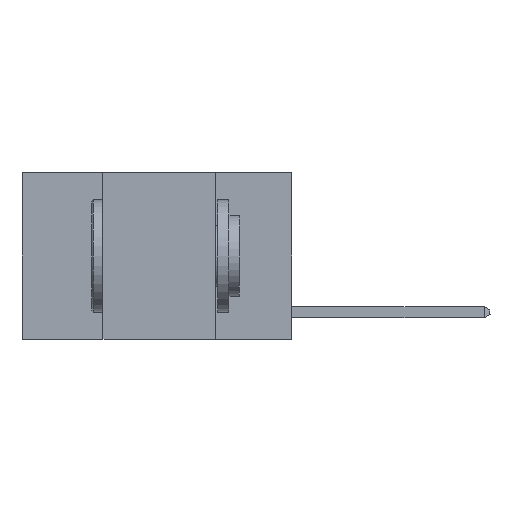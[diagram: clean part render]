
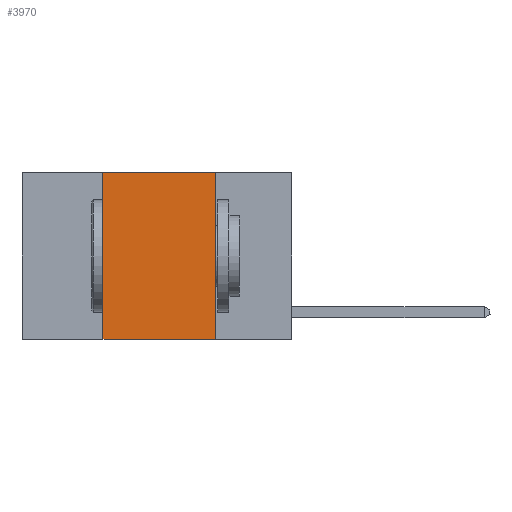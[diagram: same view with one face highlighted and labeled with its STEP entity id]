
A CAD part, left-side view. The second image highlights one B-rep face of the part: STEP entity #3970.
In plain terms, the highlighted planar face has unit normal (-1, 0, 0).
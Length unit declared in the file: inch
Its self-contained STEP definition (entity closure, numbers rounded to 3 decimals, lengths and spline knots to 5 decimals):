
#795 = VERTEX_POINT ( 'NONE', #7613 ) ;
#1009 = DIRECTION ( 'NONE',  ( 0., 0., 1. ) ) ;
#2257 = CARTESIAN_POINT ( 'NONE',  ( 0., 0.17, 0. ) ) ;
#3109 = CARTESIAN_POINT ( 'NONE',  ( 0., 0.6, 0. ) ) ;
#3128 = VERTEX_POINT ( 'NONE', #8040 ) ;
#3388 = VECTOR ( 'NONE', #11484, 39.37008 ) ;
#3541 = CARTESIAN_POINT ( 'NONE',  ( 0., 0.6, 0. ) ) ;
#3970 = ADVANCED_FACE ( 'NONE', ( #9713 ), #4510, .F. ) ;
#4170 = ORIENTED_EDGE ( 'NONE', *, *, #9298, .T. ) ;
#4510 = PLANE ( 'NONE',  #6980 ) ;
#4902 = VERTEX_POINT ( 'NONE', #6305 ) ;
#5471 = VECTOR ( 'NONE', #7393, 39.37008 ) ;
#6305 = CARTESIAN_POINT ( 'NONE',  ( 0., 0.42, 0. ) ) ;
#6980 = AXIS2_PLACEMENT_3D ( 'NONE', #3109, #11218, #14520 ) ;
#7393 = DIRECTION ( 'NONE',  ( 0., -1., 0. ) ) ;
#7411 = VECTOR ( 'NONE', #15067, 39.37008 ) ;
#7613 = CARTESIAN_POINT ( 'NONE',  ( 0., 0.17, -0.37 ) ) ;
#8040 = CARTESIAN_POINT ( 'NONE',  ( 0., 0.42, -0.37 ) ) ;
#9298 = EDGE_CURVE ( 'NONE', #3128, #795, #10453, .T. ) ;
#9713 = FACE_OUTER_BOUND ( 'NONE', #15528, .T. ) ;
#10453 = LINE ( 'NONE', #13846, #5471 ) ;
#10499 = LINE ( 'NONE', #2257, #7411 ) ;
#11218 = DIRECTION ( 'NONE',  ( 1., 0., 0. ) ) ;
#11484 = DIRECTION ( 'NONE',  ( 0., -1., 0. ) ) ;
#12625 = CARTESIAN_POINT ( 'NONE',  ( 0., 0.42, 0. ) ) ;
#13846 = CARTESIAN_POINT ( 'NONE',  ( 0., 0.6, -0.37 ) ) ;
#13991 = VERTEX_POINT ( 'NONE', #15413 ) ;
#14520 = DIRECTION ( 'NONE',  ( 0., 0., -1. ) ) ;
#15067 = DIRECTION ( 'NONE',  ( 0., 0., -1. ) ) ;
#15413 = CARTESIAN_POINT ( 'NONE',  ( 0., 0.17, 0. ) ) ;
#15528 = EDGE_LOOP ( 'NONE', ( #17459, #20319, #20149, #4170 ) ) ;
#15790 = EDGE_CURVE ( 'NONE', #13991, #795, #10499, .T. ) ;
#15887 = LINE ( 'NONE', #12625, #17120 ) ;
#16778 = LINE ( 'NONE', #3541, #3388 ) ;
#17120 = VECTOR ( 'NONE', #1009, 39.37008 ) ;
#17459 = ORIENTED_EDGE ( 'NONE', *, *, #15790, .F. ) ;
#19192 = EDGE_CURVE ( 'NONE', #4902, #13991, #16778, .T. ) ;
#19867 = EDGE_CURVE ( 'NONE', #3128, #4902, #15887, .T. ) ;
#20149 = ORIENTED_EDGE ( 'NONE', *, *, #19867, .F. ) ;
#20319 = ORIENTED_EDGE ( 'NONE', *, *, #19192, .F. ) ;
